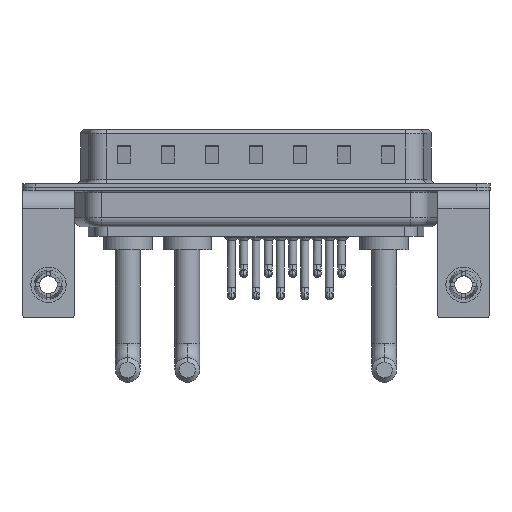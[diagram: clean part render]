
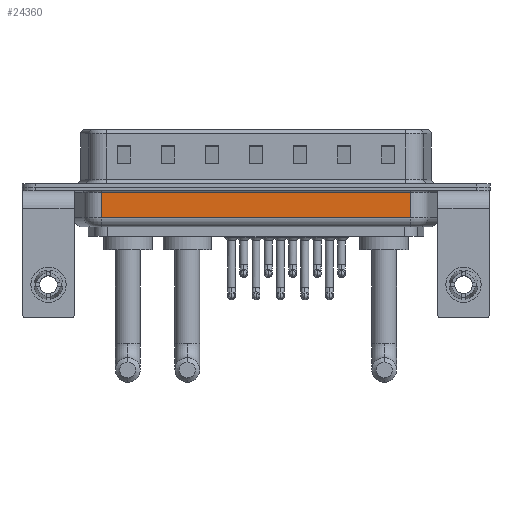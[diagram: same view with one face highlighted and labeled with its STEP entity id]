
A CAD part, front view. The second image highlights one B-rep face of the part: STEP entity #24360.
In plain terms, the highlighted planar face has unit normal (0, -1, 0).
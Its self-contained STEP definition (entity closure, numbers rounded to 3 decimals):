
#1519 = CARTESIAN_POINT ( 'NONE',  ( 41.044, -5.35, -4.5 ) ) ;
#2001 = VERTEX_POINT ( 'NONE', #13606 ) ;
#3132 = EDGE_CURVE ( 'NONE', #12573, #20935, #17040, .T. ) ;
#3247 = DIRECTION ( 'NONE',  ( 0., 0., 1. ) ) ;
#3512 = VECTOR ( 'NONE', #19218, 1000. ) ;
#3646 = EDGE_LOOP ( 'NONE', ( #14608, #25518, #22357, #4057 ) ) ;
#4057 = ORIENTED_EDGE ( 'NONE', *, *, #4980, .T. ) ;
#4081 = EDGE_CURVE ( 'NONE', #12573, #6336, #22738, .T. ) ;
#4980 = EDGE_CURVE ( 'NONE', #2001, #20935, #23048, .T. ) ;
#5082 = CARTESIAN_POINT ( 'NONE',  ( 6.006, -5.35, -4.5 ) ) ;
#5212 = PLANE ( 'NONE',  #18968 ) ;
#5521 = VECTOR ( 'NONE', #3247, 1000. ) ;
#6336 = VERTEX_POINT ( 'NONE', #9967 ) ;
#6976 = VECTOR ( 'NONE', #17547, 1000. ) ;
#7282 = LINE ( 'NONE', #1519, #6976 ) ;
#7306 = CARTESIAN_POINT ( 'NONE',  ( 6.006, -5.35, -4.5 ) ) ;
#9967 = CARTESIAN_POINT ( 'NONE',  ( 41.044, -5.35, -3.5 ) ) ;
#10064 = CARTESIAN_POINT ( 'NONE',  ( 6.006, -5.35, -3.5 ) ) ;
#11007 = FACE_OUTER_BOUND ( 'NONE', #3646, .T. ) ;
#12573 = VERTEX_POINT ( 'NONE', #10064 ) ;
#13606 = CARTESIAN_POINT ( 'NONE',  ( 41.044, -5.35, -0.65 ) ) ;
#13894 = CARTESIAN_POINT ( 'NONE',  ( 6.006, -5.35, -0.65 ) ) ;
#14608 = ORIENTED_EDGE ( 'NONE', *, *, #3132, .F. ) ;
#16906 = DIRECTION ( 'NONE',  ( 0., 1., 0. ) ) ;
#17040 = LINE ( 'NONE', #7306, #5521 ) ;
#17547 = DIRECTION ( 'NONE',  ( 0., 0., 1. ) ) ;
#18462 = EDGE_CURVE ( 'NONE', #6336, #2001, #7282, .T. ) ;
#18968 = AXIS2_PLACEMENT_3D ( 'NONE', #5082, #16906, #23343 ) ;
#19218 = DIRECTION ( 'NONE',  ( -1., 0., 0. ) ) ;
#20935 = VERTEX_POINT ( 'NONE', #13894 ) ;
#22357 = ORIENTED_EDGE ( 'NONE', *, *, #18462, .T. ) ;
#22738 = LINE ( 'NONE', #24852, #24865 ) ;
#22872 = DIRECTION ( 'NONE',  ( 1., 0., 0. ) ) ;
#23048 = LINE ( 'NONE', #23310, #3512 ) ;
#23310 = CARTESIAN_POINT ( 'NONE',  ( 6.006, -5.35, -0.65 ) ) ;
#23343 = DIRECTION ( 'NONE',  ( 0., 0., 1. ) ) ;
#24360 = ADVANCED_FACE ( 'NONE', ( #11007 ), #5212, .F. ) ;
#24852 = CARTESIAN_POINT ( 'NONE',  ( 6.006, -5.35, -3.5 ) ) ;
#24865 = VECTOR ( 'NONE', #22872, 1000. ) ;
#25518 = ORIENTED_EDGE ( 'NONE', *, *, #4081, .T. ) ;
